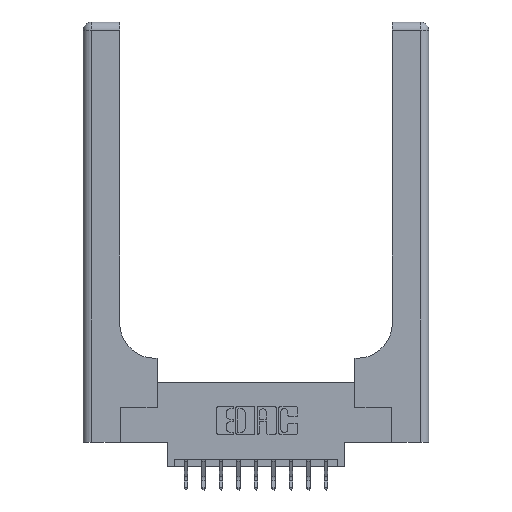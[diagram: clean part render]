
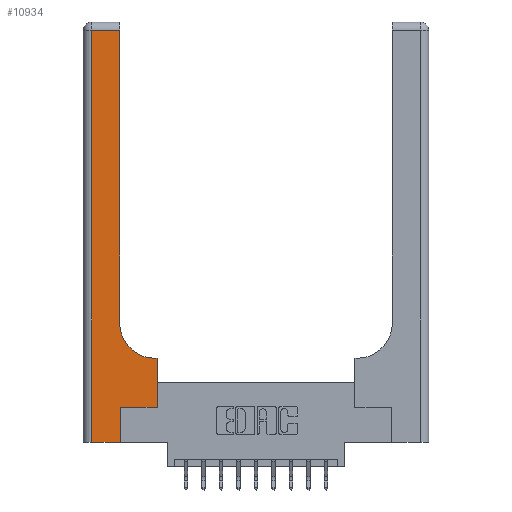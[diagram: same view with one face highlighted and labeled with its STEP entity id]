
A CAD part, top view. The second image highlights one B-rep face of the part: STEP entity #10934.
In plain terms, the highlighted planar face has unit normal (0, 0, 1).
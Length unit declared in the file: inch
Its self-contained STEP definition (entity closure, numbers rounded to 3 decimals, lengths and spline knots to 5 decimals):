
#322 = DIRECTION ( 'NONE',  ( 0., 1., 0. ) ) ;
#605 = CARTESIAN_POINT ( 'NONE',  ( 0.26, 2.94, 0.37 ) ) ;
#901 = DIRECTION ( 'NONE',  ( 1., 0., 0. ) ) ;
#1056 = EDGE_CURVE ( 'NONE', #3928, #9317, #8636, .T. ) ;
#1310 = VERTEX_POINT ( 'NONE', #6055 ) ;
#1473 = ORIENTED_EDGE ( 'NONE', *, *, #9031, .T. ) ;
#1485 = LINE ( 'NONE', #11625, #16113 ) ;
#1603 = VERTEX_POINT ( 'NONE', #6246 ) ;
#1620 = CIRCLE ( 'NONE', #13768, 0.25 ) ;
#1726 = VERTEX_POINT ( 'NONE', #14353 ) ;
#1909 = ORIENTED_EDGE ( 'NONE', *, *, #1056, .T. ) ;
#2014 = VECTOR ( 'NONE', #10360, 39.37008 ) ;
#2340 = CARTESIAN_POINT ( 'NONE',  ( 0.26, 0.6, 0.37 ) ) ;
#2854 = ORIENTED_EDGE ( 'NONE', *, *, #9782, .T. ) ;
#3333 = VERTEX_POINT ( 'NONE', #16221 ) ;
#3682 = CARTESIAN_POINT ( 'NONE',  ( 0., 3., 0.37 ) ) ;
#3928 = VERTEX_POINT ( 'NONE', #11323 ) ;
#3998 = AXIS2_PLACEMENT_3D ( 'NONE', #3682, #8735, #7883 ) ;
#4124 = CARTESIAN_POINT ( 'NONE',  ( 0.26, 3., 0.37 ) ) ;
#4546 = LINE ( 'NONE', #13540, #7250 ) ;
#4656 = ORIENTED_EDGE ( 'NONE', *, *, #7343, .T. ) ;
#5280 = VECTOR ( 'NONE', #322, 39.37008 ) ;
#5381 = DIRECTION ( 'NONE',  ( 0., 1., 0. ) ) ;
#5419 = CARTESIAN_POINT ( 'NONE',  ( 0.51, 0.85, 0.37 ) ) ;
#5435 = LINE ( 'NONE', #12838, #5280 ) ;
#5664 = DIRECTION ( 'NONE',  ( 1., 0., 0. ) ) ;
#6009 = VECTOR ( 'NONE', #901, 39.37008 ) ;
#6055 = CARTESIAN_POINT ( 'NONE',  ( 0.265, 0.25, 0.37 ) ) ;
#6143 = DIRECTION ( 'NONE',  ( -1., 0., 0. ) ) ;
#6246 = CARTESIAN_POINT ( 'NONE',  ( 0.06, 2.94, 0.37 ) ) ;
#7174 = VECTOR ( 'NONE', #5381, 39.37008 ) ;
#7250 = VECTOR ( 'NONE', #15781, 39.37008 ) ;
#7343 = EDGE_CURVE ( 'NONE', #14689, #1310, #5435, .T. ) ;
#7840 = VECTOR ( 'NONE', #9647, 39.37008 ) ;
#7883 = DIRECTION ( 'NONE',  ( -1., 0., 0. ) ) ;
#7983 = LINE ( 'NONE', #15426, #2014 ) ;
#8636 = LINE ( 'NONE', #2340, #11853 ) ;
#8735 = DIRECTION ( 'NONE',  ( 0., 0., -1. ) ) ;
#9031 = EDGE_CURVE ( 'NONE', #16223, #11608, #15465, .T. ) ;
#9317 = VERTEX_POINT ( 'NONE', #15881 ) ;
#9402 = LINE ( 'NONE', #9568, #6009 ) ;
#9568 = CARTESIAN_POINT ( 'NONE',  ( 0., 0., 0.37 ) ) ;
#9647 = DIRECTION ( 'NONE',  ( 1., 0., 0. ) ) ;
#9782 = EDGE_CURVE ( 'NONE', #1726, #3928, #1485, .T. ) ;
#9974 = FACE_OUTER_BOUND ( 'NONE', #14036, .T. ) ;
#10360 = DIRECTION ( 'NONE',  ( 0., -1., 0. ) ) ;
#10871 = LINE ( 'NONE', #15929, #7840 ) ;
#10934 = ADVANCED_FACE ( 'NONE', ( #9974 ), #15023, .F. ) ;
#10965 = EDGE_CURVE ( 'NONE', #9317, #16223, #1620, .T. ) ;
#11273 = ORIENTED_EDGE ( 'NONE', *, *, #10965, .T. ) ;
#11323 = CARTESIAN_POINT ( 'NONE',  ( 0.528, 0.6, 0.37 ) ) ;
#11608 = VERTEX_POINT ( 'NONE', #605 ) ;
#11625 = CARTESIAN_POINT ( 'NONE',  ( 0.528, 0.25, 0.37 ) ) ;
#11822 = DIRECTION ( 'NONE',  ( 0., 0., -1. ) ) ;
#11853 = VECTOR ( 'NONE', #6143, 39.37008 ) ;
#12236 = ORIENTED_EDGE ( 'NONE', *, *, #14894, .T. ) ;
#12375 = ORIENTED_EDGE ( 'NONE', *, *, #13590, .T. ) ;
#12838 = CARTESIAN_POINT ( 'NONE',  ( 0.265, 0., 0.37 ) ) ;
#13057 = ORIENTED_EDGE ( 'NONE', *, *, #13562, .T. ) ;
#13540 = CARTESIAN_POINT ( 'NONE',  ( 0., 2.94, 0.37 ) ) ;
#13562 = EDGE_CURVE ( 'NONE', #3333, #14689, #9402, .T. ) ;
#13590 = EDGE_CURVE ( 'NONE', #1310, #1726, #10871, .T. ) ;
#13768 = AXIS2_PLACEMENT_3D ( 'NONE', #5419, #11822, #5664 ) ;
#13772 = EDGE_CURVE ( 'NONE', #1603, #3333, #7983, .T. ) ;
#14028 = DIRECTION ( 'NONE',  ( 0., 1., 0. ) ) ;
#14036 = EDGE_LOOP ( 'NONE', ( #1473, #12236, #15234, #13057, #4656, #12375, #2854, #1909, #11273 ) ) ;
#14189 = CARTESIAN_POINT ( 'NONE',  ( 0.26, 0.85, 0.37 ) ) ;
#14353 = CARTESIAN_POINT ( 'NONE',  ( 0.528, 0.25, 0.37 ) ) ;
#14689 = VERTEX_POINT ( 'NONE', #16272 ) ;
#14894 = EDGE_CURVE ( 'NONE', #11608, #1603, #4546, .T. ) ;
#15023 = PLANE ( 'NONE',  #3998 ) ;
#15234 = ORIENTED_EDGE ( 'NONE', *, *, #13772, .T. ) ;
#15426 = CARTESIAN_POINT ( 'NONE',  ( 0.06, 3., 0.37 ) ) ;
#15465 = LINE ( 'NONE', #4124, #7174 ) ;
#15781 = DIRECTION ( 'NONE',  ( -1., 0., 0. ) ) ;
#15881 = CARTESIAN_POINT ( 'NONE',  ( 0.51, 0.6, 0.37 ) ) ;
#15929 = CARTESIAN_POINT ( 'NONE',  ( 0.265, 0.25, 0.37 ) ) ;
#16113 = VECTOR ( 'NONE', #14028, 39.37008 ) ;
#16221 = CARTESIAN_POINT ( 'NONE',  ( 0.06, 0., 0.37 ) ) ;
#16223 = VERTEX_POINT ( 'NONE', #14189 ) ;
#16272 = CARTESIAN_POINT ( 'NONE',  ( 0.265, 0., 0.37 ) ) ;
